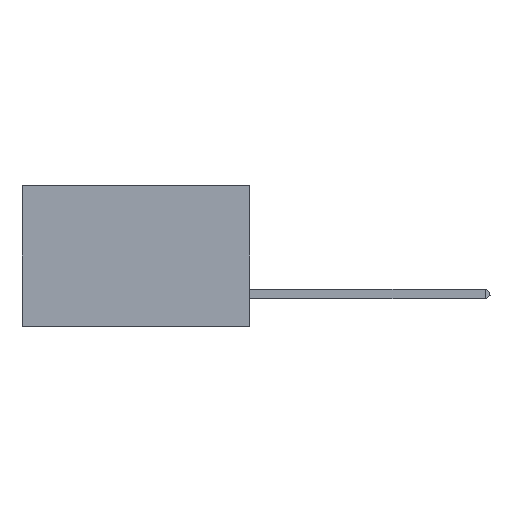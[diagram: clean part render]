
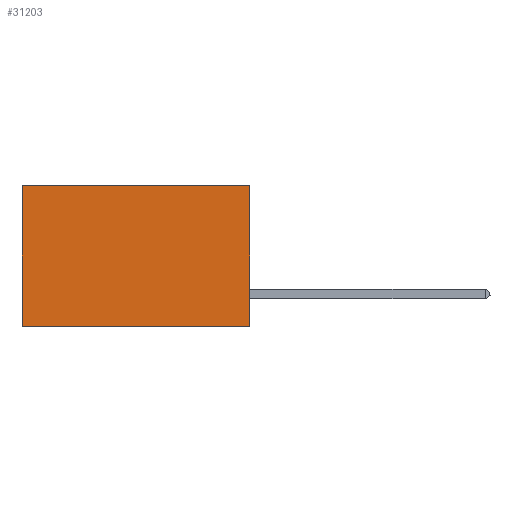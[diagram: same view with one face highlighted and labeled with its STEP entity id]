
A CAD part, left-side view. The second image highlights one B-rep face of the part: STEP entity #31203.
In plain terms, the highlighted planar face has unit normal (-1, 0, 0).
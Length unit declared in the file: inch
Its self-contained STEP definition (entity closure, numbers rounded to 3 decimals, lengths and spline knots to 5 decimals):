
#526 = ORIENTED_EDGE ( 'NONE', *, *, #20466, .F. ) ;
#748 = EDGE_CURVE ( 'NONE', #18991, #1019, #6408, .T. ) ;
#1019 = VERTEX_POINT ( 'NONE', #15140 ) ;
#1631 = FACE_OUTER_BOUND ( 'NONE', #14954, .T. ) ;
#2254 = CARTESIAN_POINT ( 'NONE',  ( 0.2875, 0., 0. ) ) ;
#4115 = CARTESIAN_POINT ( 'NONE',  ( 0.2875, 0.6, 0. ) ) ;
#5981 = CARTESIAN_POINT ( 'NONE',  ( 0.2875, 0.6, 0. ) ) ;
#6043 = CARTESIAN_POINT ( 'NONE',  ( 0.2875, 0., -0.37 ) ) ;
#6408 = LINE ( 'NONE', #4115, #18805 ) ;
#7087 = CARTESIAN_POINT ( 'NONE',  ( 0.2875, 0., -0.37 ) ) ;
#7384 = ORIENTED_EDGE ( 'NONE', *, *, #31388, .T. ) ;
#7542 = DIRECTION ( 'NONE',  ( 1., 0., 0. ) ) ;
#9724 = VERTEX_POINT ( 'NONE', #6043 ) ;
#10553 = VECTOR ( 'NONE', #29756, 39.37008 ) ;
#11721 = CARTESIAN_POINT ( 'NONE',  ( 0.2875, 0., 0. ) ) ;
#13506 = DIRECTION ( 'NONE',  ( 0., 1., 0. ) ) ;
#14090 = DIRECTION ( 'NONE',  ( 0., 0., -1. ) ) ;
#14221 = ORIENTED_EDGE ( 'NONE', *, *, #748, .T. ) ;
#14626 = DIRECTION ( 'NONE',  ( 0., 0., -1. ) ) ;
#14954 = EDGE_LOOP ( 'NONE', ( #14221, #526, #23428, #7384 ) ) ;
#15140 = CARTESIAN_POINT ( 'NONE',  ( 0.2875, 0.6, -0.37 ) ) ;
#17851 = LINE ( 'NONE', #25638, #28244 ) ;
#18248 = VECTOR ( 'NONE', #19211, 39.37008 ) ;
#18805 = VECTOR ( 'NONE', #14090, 39.37008 ) ;
#18991 = VERTEX_POINT ( 'NONE', #5981 ) ;
#19211 = DIRECTION ( 'NONE',  ( 0., 1., 0. ) ) ;
#20188 = LINE ( 'NONE', #23466, #10553 ) ;
#20466 = EDGE_CURVE ( 'NONE', #9724, #1019, #29354, .T. ) ;
#22336 = PLANE ( 'NONE',  #28156 ) ;
#22957 = VERTEX_POINT ( 'NONE', #11721 ) ;
#23428 = ORIENTED_EDGE ( 'NONE', *, *, #30988, .F. ) ;
#23466 = CARTESIAN_POINT ( 'NONE',  ( 0.2875, 0., 0. ) ) ;
#25638 = CARTESIAN_POINT ( 'NONE',  ( 0.2875, 0., 0. ) ) ;
#28156 = AXIS2_PLACEMENT_3D ( 'NONE', #2254, #7542, #14626 ) ;
#28244 = VECTOR ( 'NONE', #13506, 39.37008 ) ;
#29354 = LINE ( 'NONE', #7087, #18248 ) ;
#29756 = DIRECTION ( 'NONE',  ( 0., 0., -1. ) ) ;
#30988 = EDGE_CURVE ( 'NONE', #22957, #9724, #20188, .T. ) ;
#31203 = ADVANCED_FACE ( 'NONE', ( #1631 ), #22336, .F. ) ;
#31388 = EDGE_CURVE ( 'NONE', #22957, #18991, #17851, .T. ) ;
